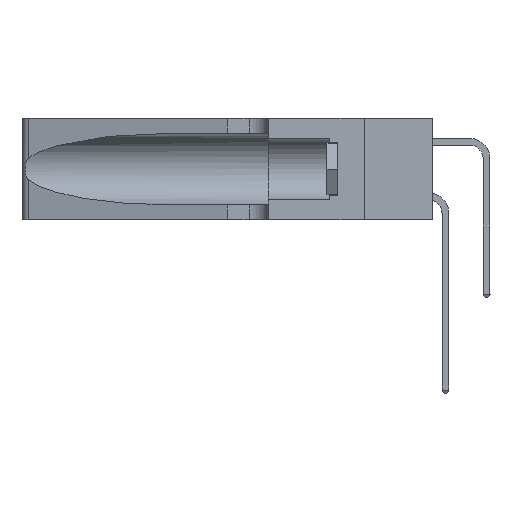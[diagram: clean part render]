
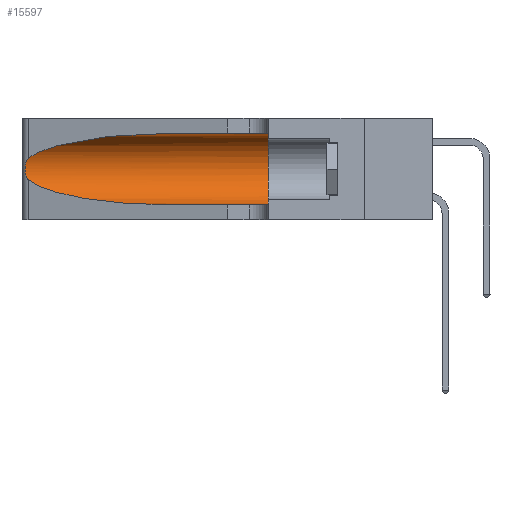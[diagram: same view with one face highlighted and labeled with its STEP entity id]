
A CAD part, left-side view. The second image highlights one B-rep face of the part: STEP entity #15597.
In plain terms, the highlighted cylindrical face has radius 3.308 mm (diameter 6.617 mm), a partial arc.
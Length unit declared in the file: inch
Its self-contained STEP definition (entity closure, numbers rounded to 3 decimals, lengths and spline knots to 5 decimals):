
#340 =( BOUNDED_CURVE ( )  B_SPLINE_CURVE ( 3, ( #6471, #18896, #8051, #11467 ),
 .UNSPECIFIED., .F., .F. ) 
 B_SPLINE_CURVE_WITH_KNOTS ( ( 4, 4 ),
 ( 3.44316, 4.71239 ),
 .UNSPECIFIED. ) 
 CURVE ( )  GEOMETRIC_REPRESENTATION_ITEM ( )  RATIONAL_B_SPLINE_CURVE ( ( 1., 0.87, 0.87, 1. ) ) 
 REPRESENTATION_ITEM ( '' )  );
#733 = CARTESIAN_POINT ( 'NONE',  ( 0.1305, 0.72297, 0.31525 ) ) ;
#1026 = CARTESIAN_POINT ( 'NONE',  ( 0.25487, 1.22718, 0.14631 ) ) ;
#1335 = CARTESIAN_POINT ( 'NONE',  ( 0.18966, 0.96281, 0.31525 ) ) ;
#1838 = LINE ( 'NONE', #3741, #7716 ) ;
#2237 = ORIENTED_EDGE ( 'NONE', *, *, #21864, .T. ) ;
#3741 = CARTESIAN_POINT ( 'NONE',  ( 0.1305, 1.61858, 0.05475 ) ) ;
#3829 = VERTEX_POINT ( 'NONE', #22082 ) ;
#4181 = EDGE_CURVE ( 'NONE', #11096, #12558, #14254, .T. ) ;
#4784 = B_SPLINE_CURVE_WITH_KNOTS ( 'NONE', 3,
 ( #13262, #18834, #16956, #22485, #22646, #9936, #22417, #6483, #17115, #8062, #13569, #22569, #6253, #1026 ),
 .UNSPECIFIED., .F., .F.,
 ( 4, 2, 2, 2, 2, 2, 4 ),
 ( 0., 0.00027, 0.00053, 0.00107, 0.0016, 0.00187, 0.00214 ),
 .UNSPECIFIED. ) ;
#5465 = CARTESIAN_POINT ( 'NONE',  ( 0.1305, 0.35, 0.185 ) ) ;
#5707 = DIRECTION ( 'NONE',  ( 0., -1., 0. ) ) ;
#6253 = CARTESIAN_POINT ( 'NONE',  ( 0.25555, 1.22993, 0.14849 ) ) ;
#6377 = VERTEX_POINT ( 'NONE', #7043 ) ;
#6385 = ORIENTED_EDGE ( 'NONE', *, *, #10906, .T. ) ;
#6471 = CARTESIAN_POINT ( 'NONE',  ( 0.25487, 1.22718, 0.14631 ) ) ;
#6483 = CARTESIAN_POINT ( 'NONE',  ( 0.26075, 1.23896, 0.178 ) ) ;
#6575 = CARTESIAN_POINT ( 'NONE',  ( 0.1305, 0.72297, 0.31525 ) ) ;
#6867 = CARTESIAN_POINT ( 'NONE',  ( 0.25487, 1.22718, 0.22369 ) ) ;
#7043 = CARTESIAN_POINT ( 'NONE',  ( 0.25487, 1.22718, 0.14631 ) ) ;
#7069 = VERTEX_POINT ( 'NONE', #14461 ) ;
#7261 = DIRECTION ( 'NONE',  ( 0., 1., 0. ) ) ;
#7525 = AXIS2_PLACEMENT_3D ( 'NONE', #5465, #7261, #14057 ) ;
#7716 = VECTOR ( 'NONE', #5707, 39.37008 ) ;
#8051 = CARTESIAN_POINT ( 'NONE',  ( 0.18966, 0.96281, 0.05475 ) ) ;
#8062 = CARTESIAN_POINT ( 'NONE',  ( 0.25856, 1.23593, 0.16098 ) ) ;
#9840 = EDGE_LOOP ( 'NONE', ( #6385, #19286, #2237, #11226, #12310, #10031 ) ) ;
#9936 = CARTESIAN_POINT ( 'NONE',  ( 0.26018, 1.23835, 0.19895 ) ) ;
#10031 = ORIENTED_EDGE ( 'NONE', *, *, #4181, .F. ) ;
#10443 = CYLINDRICAL_SURFACE ( 'NONE', #17401, 0.13025 ) ;
#10906 = EDGE_CURVE ( 'NONE', #11096, #3829, #13067, .T. ) ;
#11096 = VERTEX_POINT ( 'NONE', #733 ) ;
#11226 = ORIENTED_EDGE ( 'NONE', *, *, #21541, .T. ) ;
#11467 = CARTESIAN_POINT ( 'NONE',  ( 0.1305, 0.72297, 0.05475 ) ) ;
#12310 = ORIENTED_EDGE ( 'NONE', *, *, #14077, .F. ) ;
#12558 = VERTEX_POINT ( 'NONE', #18207 ) ;
#13067 =( BOUNDED_CURVE ( )  B_SPLINE_CURVE ( 3, ( #6575, #1335, #15615, #6867 ),
 .UNSPECIFIED., .F., .T. ) 
 B_SPLINE_CURVE_WITH_KNOTS ( ( 4, 4 ),
 ( 1.5708, 2.84003 ),
 .UNSPECIFIED. ) 
 CURVE ( )  GEOMETRIC_REPRESENTATION_ITEM ( )  RATIONAL_B_SPLINE_CURVE ( ( 1., 0.87, 0.87, 1. ) ) 
 REPRESENTATION_ITEM ( '' )  );
#13262 = CARTESIAN_POINT ( 'NONE',  ( 0.25487, 1.22718, 0.22369 ) ) ;
#13569 = CARTESIAN_POINT ( 'NONE',  ( 0.25789, 1.23486, 0.15765 ) ) ;
#13822 = DIRECTION ( 'NONE',  ( 0., -1., 0. ) ) ;
#14057 = DIRECTION ( 'NONE',  ( 0., 0., 1. ) ) ;
#14059 = CARTESIAN_POINT ( 'NONE',  ( 0.1305, 1.61858, 0.185 ) ) ;
#14077 = EDGE_CURVE ( 'NONE', #12558, #7069, #22820, .T. ) ;
#14254 = LINE ( 'NONE', #19132, #20159 ) ;
#14461 = CARTESIAN_POINT ( 'NONE',  ( 0.1305, 0.35, 0.05475 ) ) ;
#15597 = ADVANCED_FACE ( 'NONE', ( #17989 ), #10443, .F. ) ;
#15615 = CARTESIAN_POINT ( 'NONE',  ( 0.2373, 1.15595, 0.28018 ) ) ;
#16956 = CARTESIAN_POINT ( 'NONE',  ( 0.25639, 1.23184, 0.21858 ) ) ;
#17115 = CARTESIAN_POINT ( 'NONE',  ( 0.26017, 1.23833, 0.17102 ) ) ;
#17401 = AXIS2_PLACEMENT_3D ( 'NONE', #14059, #13822, #23046 ) ;
#17989 = FACE_OUTER_BOUND ( 'NONE', #9840, .T. ) ;
#18044 = EDGE_CURVE ( 'NONE', #3829, #6377, #4784, .T. ) ;
#18207 = CARTESIAN_POINT ( 'NONE',  ( 0.1305, 0.35, 0.31525 ) ) ;
#18834 = CARTESIAN_POINT ( 'NONE',  ( 0.25555, 1.22994, 0.2215 ) ) ;
#18896 = CARTESIAN_POINT ( 'NONE',  ( 0.2373, 1.15595, 0.08982 ) ) ;
#19132 = CARTESIAN_POINT ( 'NONE',  ( 0.1305, 1.61858, 0.31525 ) ) ;
#19286 = ORIENTED_EDGE ( 'NONE', *, *, #18044, .T. ) ;
#19921 = VERTEX_POINT ( 'NONE', #22221 ) ;
#20159 = VECTOR ( 'NONE', #21171, 39.37008 ) ;
#21171 = DIRECTION ( 'NONE',  ( 0., -1., 0. ) ) ;
#21541 = EDGE_CURVE ( 'NONE', #19921, #7069, #1838, .T. ) ;
#21864 = EDGE_CURVE ( 'NONE', #6377, #19921, #340, .T. ) ;
#22082 = CARTESIAN_POINT ( 'NONE',  ( 0.25487, 1.22718, 0.22369 ) ) ;
#22221 = CARTESIAN_POINT ( 'NONE',  ( 0.1305, 0.72297, 0.05475 ) ) ;
#22417 = CARTESIAN_POINT ( 'NONE',  ( 0.26075, 1.23896, 0.19203 ) ) ;
#22485 = CARTESIAN_POINT ( 'NONE',  ( 0.25787, 1.23484, 0.2124 ) ) ;
#22569 = CARTESIAN_POINT ( 'NONE',  ( 0.25639, 1.23186, 0.15144 ) ) ;
#22646 = CARTESIAN_POINT ( 'NONE',  ( 0.25854, 1.2359, 0.20912 ) ) ;
#22820 = CIRCLE ( 'NONE', #7525, 0.13025 ) ;
#23046 = DIRECTION ( 'NONE',  ( 0., 0., -1. ) ) ;
